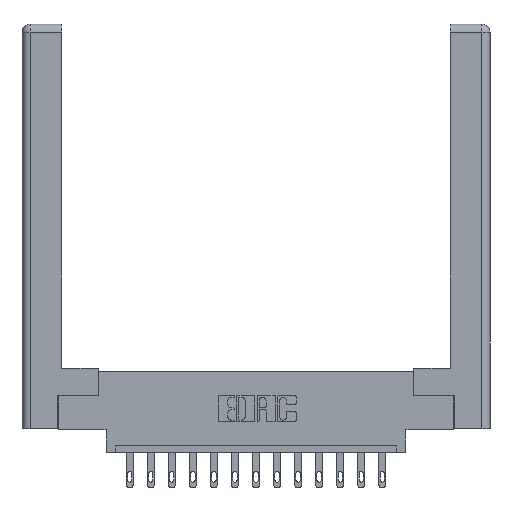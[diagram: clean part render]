
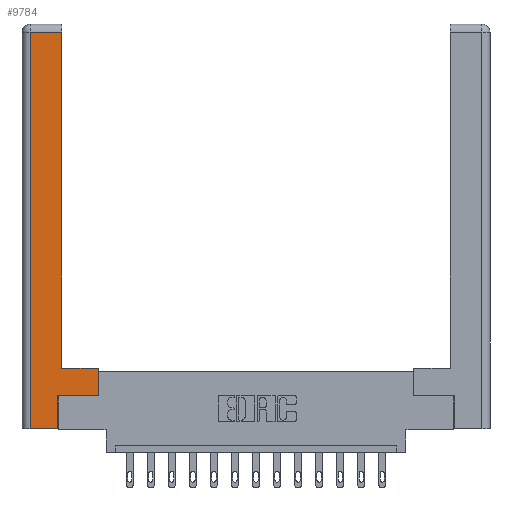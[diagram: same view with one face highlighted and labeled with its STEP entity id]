
A CAD part, top view. The second image highlights one B-rep face of the part: STEP entity #9784.
In plain terms, the highlighted planar face has unit normal (0, 0, 1).
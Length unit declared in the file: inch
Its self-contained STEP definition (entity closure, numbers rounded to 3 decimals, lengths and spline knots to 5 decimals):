
#207 = CARTESIAN_POINT ( 'NONE',  ( 0.265, 0., 0. ) ) ;
#400 = VECTOR ( 'NONE', #9262, 39.37008 ) ;
#448 = CARTESIAN_POINT ( 'NONE',  ( 0.295, 0.45, 0. ) ) ;
#482 = CARTESIAN_POINT ( 'NONE',  ( 0.565, 0.45, 0. ) ) ;
#484 = LINE ( 'NONE', #448, #5525 ) ;
#699 = VERTEX_POINT ( 'NONE', #7047 ) ;
#831 = LINE ( 'NONE', #4459, #5481 ) ;
#1061 = VECTOR ( 'NONE', #11657, 39.37008 ) ;
#1222 = EDGE_CURVE ( 'NONE', #1784, #3150, #4382, .T. ) ;
#1625 = LINE ( 'NONE', #11526, #3594 ) ;
#1784 = VERTEX_POINT ( 'NONE', #14452 ) ;
#1907 = LINE ( 'NONE', #482, #5781 ) ;
#1995 = VERTEX_POINT ( 'NONE', #15275 ) ;
#2073 = EDGE_CURVE ( 'NONE', #699, #1995, #831, .T. ) ;
#2351 = CARTESIAN_POINT ( 'NONE',  ( 0.295, 0.45, 0. ) ) ;
#2632 = EDGE_LOOP ( 'NONE', ( #13825, #10680, #2951, #14486, #5717, #7897, #3417, #5691 ) ) ;
#2951 = ORIENTED_EDGE ( 'NONE', *, *, #2073, .T. ) ;
#3150 = VERTEX_POINT ( 'NONE', #10647 ) ;
#3417 = ORIENTED_EDGE ( 'NONE', *, *, #10985, .T. ) ;
#3594 = VECTOR ( 'NONE', #5369, 39.37008 ) ;
#3982 = DIRECTION ( 'NONE',  ( 0., 1., 0. ) ) ;
#4382 = LINE ( 'NONE', #6699, #1061 ) ;
#4459 = CARTESIAN_POINT ( 'NONE',  ( 0.0615, 0., 0. ) ) ;
#4688 = VERTEX_POINT ( 'NONE', #2351 ) ;
#5369 = DIRECTION ( 'NONE',  ( 1., 0., 0. ) ) ;
#5372 = DIRECTION ( 'NONE',  ( 0., 1., 0. ) ) ;
#5481 = VECTOR ( 'NONE', #5675, 39.37008 ) ;
#5525 = VECTOR ( 'NONE', #6590, 39.37008 ) ;
#5675 = DIRECTION ( 'NONE',  ( 0., -1., 0. ) ) ;
#5691 = ORIENTED_EDGE ( 'NONE', *, *, #15649, .T. ) ;
#5717 = ORIENTED_EDGE ( 'NONE', *, *, #16063, .T. ) ;
#5781 = VECTOR ( 'NONE', #5372, 39.37008 ) ;
#5873 = VERTEX_POINT ( 'NONE', #13933 ) ;
#5893 = AXIS2_PLACEMENT_3D ( 'NONE', #14658, #6977, #5932 ) ;
#5932 = DIRECTION ( 'NONE',  ( -1., 0., 0. ) ) ;
#6026 = FACE_OUTER_BOUND ( 'NONE', #2632, .T. ) ;
#6116 = EDGE_CURVE ( 'NONE', #5873, #699, #12997, .T. ) ;
#6590 = DIRECTION ( 'NONE',  ( -1., 0., 0. ) ) ;
#6699 = CARTESIAN_POINT ( 'NONE',  ( 0.565, 0.245, 0. ) ) ;
#6977 = DIRECTION ( 'NONE',  ( 0., 0., -1. ) ) ;
#6986 = EDGE_CURVE ( 'NONE', #1995, #14221, #1625, .T. ) ;
#7047 = CARTESIAN_POINT ( 'NONE',  ( 0.0615, 2.94, 0. ) ) ;
#7897 = ORIENTED_EDGE ( 'NONE', *, *, #1222, .T. ) ;
#8652 = VECTOR ( 'NONE', #3982, 39.37008 ) ;
#8657 = EDGE_CURVE ( 'NONE', #4688, #5873, #14816, .T. ) ;
#9262 = DIRECTION ( 'NONE',  ( 0., 1., 0. ) ) ;
#9419 = CARTESIAN_POINT ( 'NONE',  ( 0.565, 0.45, 0. ) ) ;
#9516 = PLANE ( 'NONE',  #5893 ) ;
#9784 = ADVANCED_FACE ( 'NONE', ( #6026 ), #9516, .F. ) ;
#10180 = CARTESIAN_POINT ( 'NONE',  ( 0.265, 0.245, 0. ) ) ;
#10605 = CARTESIAN_POINT ( 'NONE',  ( 0.0615, 2.94, 0. ) ) ;
#10647 = CARTESIAN_POINT ( 'NONE',  ( 0.565, 0.245, 0. ) ) ;
#10680 = ORIENTED_EDGE ( 'NONE', *, *, #6116, .T. ) ;
#10985 = EDGE_CURVE ( 'NONE', #3150, #15019, #1907, .T. ) ;
#11526 = CARTESIAN_POINT ( 'NONE',  ( 0.265, 0., 0. ) ) ;
#11657 = DIRECTION ( 'NONE',  ( 1., 0., 0. ) ) ;
#12988 = VECTOR ( 'NONE', #15600, 39.37008 ) ;
#12997 = LINE ( 'NONE', #10605, #12988 ) ;
#13034 = CARTESIAN_POINT ( 'NONE',  ( 0.295, 3., 0. ) ) ;
#13825 = ORIENTED_EDGE ( 'NONE', *, *, #8657, .T. ) ;
#13933 = CARTESIAN_POINT ( 'NONE',  ( 0.295, 2.94, 0. ) ) ;
#14108 = LINE ( 'NONE', #10180, #8652 ) ;
#14221 = VERTEX_POINT ( 'NONE', #207 ) ;
#14452 = CARTESIAN_POINT ( 'NONE',  ( 0.265, 0.245, 0. ) ) ;
#14486 = ORIENTED_EDGE ( 'NONE', *, *, #6986, .T. ) ;
#14658 = CARTESIAN_POINT ( 'NONE',  ( 0., 0., 0. ) ) ;
#14816 = LINE ( 'NONE', #13034, #400 ) ;
#15019 = VERTEX_POINT ( 'NONE', #9419 ) ;
#15275 = CARTESIAN_POINT ( 'NONE',  ( 0.0615, 0., 0. ) ) ;
#15600 = DIRECTION ( 'NONE',  ( -1., 0., 0. ) ) ;
#15649 = EDGE_CURVE ( 'NONE', #15019, #4688, #484, .T. ) ;
#16063 = EDGE_CURVE ( 'NONE', #14221, #1784, #14108, .T. ) ;
